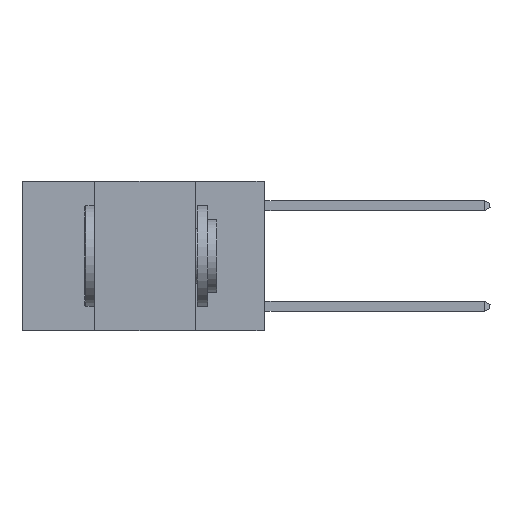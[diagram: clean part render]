
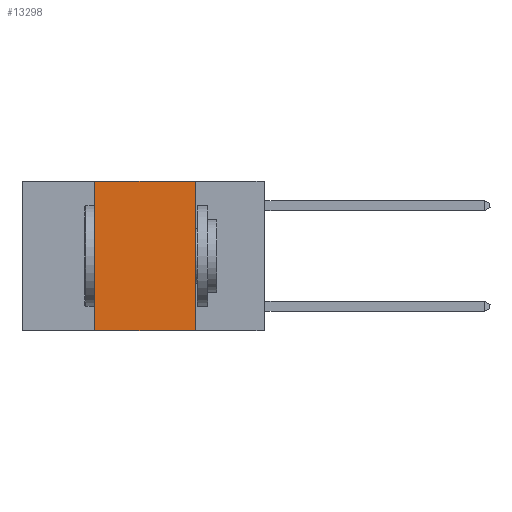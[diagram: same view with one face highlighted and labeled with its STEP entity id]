
A CAD part, left-side view. The second image highlights one B-rep face of the part: STEP entity #13298.
In plain terms, the highlighted planar face has unit normal (-1, 0, 0).
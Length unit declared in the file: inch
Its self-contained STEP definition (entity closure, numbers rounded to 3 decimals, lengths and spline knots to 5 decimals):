
#95 = EDGE_CURVE ( 'NONE', #1592, #16498, #669, .T. ) ;
#669 = LINE ( 'NONE', #16622, #11893 ) ;
#747 = LINE ( 'NONE', #9930, #14220 ) ;
#1431 = FACE_OUTER_BOUND ( 'NONE', #25225, .T. ) ;
#1592 = VERTEX_POINT ( 'NONE', #19608 ) ;
#1893 = LINE ( 'NONE', #8829, #3598 ) ;
#3598 = VECTOR ( 'NONE', #15441, 39.37008 ) ;
#5084 = ORIENTED_EDGE ( 'NONE', *, *, #14743, .F. ) ;
#5632 = CARTESIAN_POINT ( 'NONE',  ( 0., 0.17, -0.37 ) ) ;
#8149 = ORIENTED_EDGE ( 'NONE', *, *, #18153, .T. ) ;
#8829 = CARTESIAN_POINT ( 'NONE',  ( 0., 0.17, 0. ) ) ;
#8998 = ORIENTED_EDGE ( 'NONE', *, *, #16954, .F. ) ;
#9906 = CARTESIAN_POINT ( 'NONE',  ( 0., 0.17, 0. ) ) ;
#9930 = CARTESIAN_POINT ( 'NONE',  ( 0., 0.6, -0.37 ) ) ;
#9999 = DIRECTION ( 'NONE',  ( 0., 0., 1. ) ) ;
#10123 = VERTEX_POINT ( 'NONE', #5632 ) ;
#10378 = VERTEX_POINT ( 'NONE', #9906 ) ;
#11718 = AXIS2_PLACEMENT_3D ( 'NONE', #18112, #29537, #25044 ) ;
#11893 = VECTOR ( 'NONE', #9999, 39.37008 ) ;
#13119 = CARTESIAN_POINT ( 'NONE',  ( 0., 0.42, 0. ) ) ;
#13298 = ADVANCED_FACE ( 'NONE', ( #1431 ), #13910, .F. ) ;
#13910 = PLANE ( 'NONE',  #11718 ) ;
#14011 = DIRECTION ( 'NONE',  ( 0., -1., 0. ) ) ;
#14220 = VECTOR ( 'NONE', #14011, 39.37008 ) ;
#14743 = EDGE_CURVE ( 'NONE', #16498, #10378, #18295, .T. ) ;
#15441 = DIRECTION ( 'NONE',  ( 0., 0., -1. ) ) ;
#16498 = VERTEX_POINT ( 'NONE', #13119 ) ;
#16622 = CARTESIAN_POINT ( 'NONE',  ( 0., 0.42, 0. ) ) ;
#16954 = EDGE_CURVE ( 'NONE', #10378, #10123, #1893, .T. ) ;
#18112 = CARTESIAN_POINT ( 'NONE',  ( 0., 0.6, 0. ) ) ;
#18153 = EDGE_CURVE ( 'NONE', #1592, #10123, #747, .T. ) ;
#18295 = LINE ( 'NONE', #22536, #26584 ) ;
#19608 = CARTESIAN_POINT ( 'NONE',  ( 0., 0.42, -0.37 ) ) ;
#22536 = CARTESIAN_POINT ( 'NONE',  ( 0., 0.6, 0. ) ) ;
#25044 = DIRECTION ( 'NONE',  ( 0., 0., -1. ) ) ;
#25225 = EDGE_LOOP ( 'NONE', ( #8998, #5084, #26626, #8149 ) ) ;
#26584 = VECTOR ( 'NONE', #27483, 39.37008 ) ;
#26626 = ORIENTED_EDGE ( 'NONE', *, *, #95, .F. ) ;
#27483 = DIRECTION ( 'NONE',  ( 0., -1., 0. ) ) ;
#29537 = DIRECTION ( 'NONE',  ( 1., 0., 0. ) ) ;
